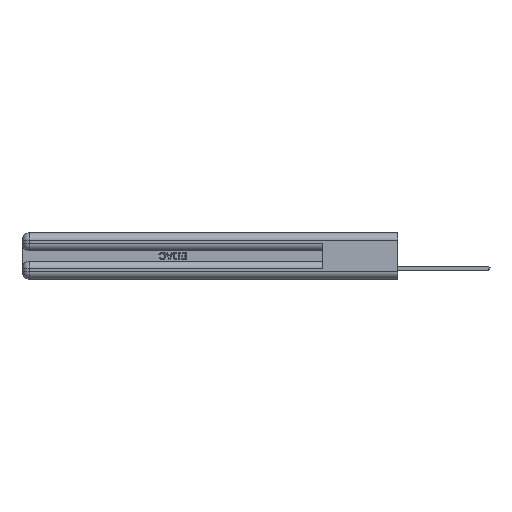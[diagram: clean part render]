
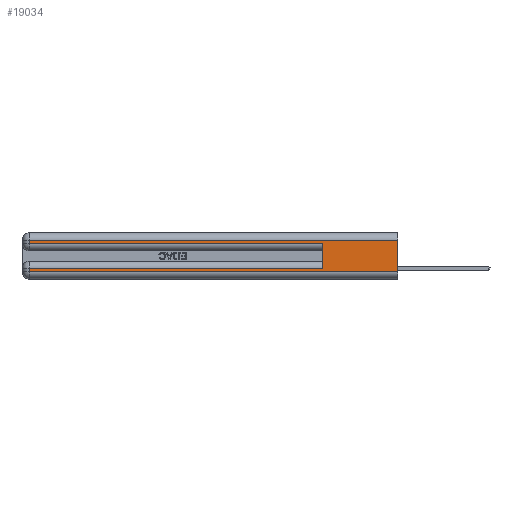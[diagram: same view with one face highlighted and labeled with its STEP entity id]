
A CAD part, left-side view. The second image highlights one B-rep face of the part: STEP entity #19034.
In plain terms, the highlighted planar face has unit normal (-1, 0, 0).
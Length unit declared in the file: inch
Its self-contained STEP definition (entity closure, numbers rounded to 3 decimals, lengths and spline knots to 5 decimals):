
#990 = CARTESIAN_POINT ( 'NONE',  ( 0., 2.94, 0.31 ) ) ;
#1127 = DIRECTION ( 'NONE',  ( 0., 1., 0. ) ) ;
#1588 = DIRECTION ( 'NONE',  ( 0., 0., -1. ) ) ;
#1990 = ORIENTED_EDGE ( 'NONE', *, *, #32443, .T. ) ;
#2297 = CARTESIAN_POINT ( 'NONE',  ( 0., 2.94, 0.06 ) ) ;
#2445 = CARTESIAN_POINT ( 'NONE',  ( 0., 0.6, 0.285 ) ) ;
#3709 = ORIENTED_EDGE ( 'NONE', *, *, #39863, .T. ) ;
#5168 = DIRECTION ( 'NONE',  ( 1., 0., 0. ) ) ;
#5198 = EDGE_CURVE ( 'NONE', #11258, #40665, #8529, .T. ) ;
#6116 = CARTESIAN_POINT ( 'NONE',  ( 0., 0.6, 0.085 ) ) ;
#6288 = LINE ( 'NONE', #39557, #42760 ) ;
#6545 = CARTESIAN_POINT ( 'NONE',  ( 0., 0.6, 0.145 ) ) ;
#6827 = VERTEX_POINT ( 'NONE', #13701 ) ;
#7124 = VECTOR ( 'NONE', #35057, 39.37008 ) ;
#8146 = CARTESIAN_POINT ( 'NONE',  ( 0., 0., 0.37 ) ) ;
#8529 = LINE ( 'NONE', #23728, #45628 ) ;
#9302 = EDGE_CURVE ( 'NONE', #11184, #38939, #22730, .T. ) ;
#10993 = VECTOR ( 'NONE', #30961, 39.37008 ) ;
#11184 = VERTEX_POINT ( 'NONE', #6116 ) ;
#11258 = VERTEX_POINT ( 'NONE', #43188 ) ;
#11453 = EDGE_CURVE ( 'NONE', #34951, #16345, #12482, .T. ) ;
#11742 = PLANE ( 'NONE',  #19495 ) ;
#12482 = LINE ( 'NONE', #37076, #37716 ) ;
#12854 = ORIENTED_EDGE ( 'NONE', *, *, #40824, .T. ) ;
#13613 = ORIENTED_EDGE ( 'NONE', *, *, #9302, .F. ) ;
#13701 = CARTESIAN_POINT ( 'NONE',  ( 0., 2.94, 0.285 ) ) ;
#14372 = LINE ( 'NONE', #19810, #10993 ) ;
#15607 = EDGE_CURVE ( 'NONE', #26946, #6827, #22947, .T. ) ;
#16345 = VERTEX_POINT ( 'NONE', #44759 ) ;
#17275 = LINE ( 'NONE', #21265, #20030 ) ;
#17277 = ORIENTED_EDGE ( 'NONE', *, *, #11453, .F. ) ;
#18064 = DIRECTION ( 'NONE',  ( 0., -1., 0. ) ) ;
#19034 = ADVANCED_FACE ( 'NONE', ( #31313 ), #11742, .F. ) ;
#19495 = AXIS2_PLACEMENT_3D ( 'NONE', #8146, #5168, #38441 ) ;
#19810 = CARTESIAN_POINT ( 'NONE',  ( 0., 0., 0.06 ) ) ;
#20030 = VECTOR ( 'NONE', #25288, 39.37008 ) ;
#20141 = CARTESIAN_POINT ( 'NONE',  ( 0., 2.94, 0.37 ) ) ;
#21265 = CARTESIAN_POINT ( 'NONE',  ( 0., 0., 0.085 ) ) ;
#21596 = CARTESIAN_POINT ( 'NONE',  ( 0., 0., 0.31 ) ) ;
#22730 = LINE ( 'NONE', #6545, #7124 ) ;
#22947 = LINE ( 'NONE', #20141, #30831 ) ;
#23545 = ORIENTED_EDGE ( 'NONE', *, *, #15607, .T. ) ;
#23566 = DIRECTION ( 'NONE',  ( 0., 0., -1. ) ) ;
#23728 = CARTESIAN_POINT ( 'NONE',  ( 0., 2.94, 0.37 ) ) ;
#25288 = DIRECTION ( 'NONE',  ( 0., 1., 0. ) ) ;
#26946 = VERTEX_POINT ( 'NONE', #990 ) ;
#28043 = EDGE_LOOP ( 'NONE', ( #17277, #3709, #23545, #1990, #13613, #12854, #33626, #40429 ) ) ;
#29167 = LINE ( 'NONE', #37458, #40372 ) ;
#30831 = VECTOR ( 'NONE', #33733, 39.37008 ) ;
#30961 = DIRECTION ( 'NONE',  ( 0., -1., 0. ) ) ;
#31313 = FACE_OUTER_BOUND ( 'NONE', #28043, .T. ) ;
#32443 = EDGE_CURVE ( 'NONE', #6827, #38939, #6288, .T. ) ;
#33626 = ORIENTED_EDGE ( 'NONE', *, *, #5198, .T. ) ;
#33733 = DIRECTION ( 'NONE',  ( 0., 0., -1. ) ) ;
#34951 = VERTEX_POINT ( 'NONE', #21596 ) ;
#35057 = DIRECTION ( 'NONE',  ( 0., 0., 1. ) ) ;
#36251 = EDGE_CURVE ( 'NONE', #40665, #16345, #14372, .T. ) ;
#37076 = CARTESIAN_POINT ( 'NONE',  ( 0., 0., 0.37 ) ) ;
#37458 = CARTESIAN_POINT ( 'NONE',  ( 0., 0., 0.31 ) ) ;
#37716 = VECTOR ( 'NONE', #1588, 39.37008 ) ;
#38441 = DIRECTION ( 'NONE',  ( 0., 0., -1. ) ) ;
#38939 = VERTEX_POINT ( 'NONE', #2445 ) ;
#39557 = CARTESIAN_POINT ( 'NONE',  ( 0., 0., 0.285 ) ) ;
#39863 = EDGE_CURVE ( 'NONE', #34951, #26946, #29167, .T. ) ;
#40372 = VECTOR ( 'NONE', #1127, 39.37008 ) ;
#40429 = ORIENTED_EDGE ( 'NONE', *, *, #36251, .T. ) ;
#40665 = VERTEX_POINT ( 'NONE', #2297 ) ;
#40824 = EDGE_CURVE ( 'NONE', #11184, #11258, #17275, .T. ) ;
#42760 = VECTOR ( 'NONE', #18064, 39.37008 ) ;
#43188 = CARTESIAN_POINT ( 'NONE',  ( 0., 2.94, 0.085 ) ) ;
#44759 = CARTESIAN_POINT ( 'NONE',  ( 0., 0., 0.06 ) ) ;
#45628 = VECTOR ( 'NONE', #23566, 39.37008 ) ;
